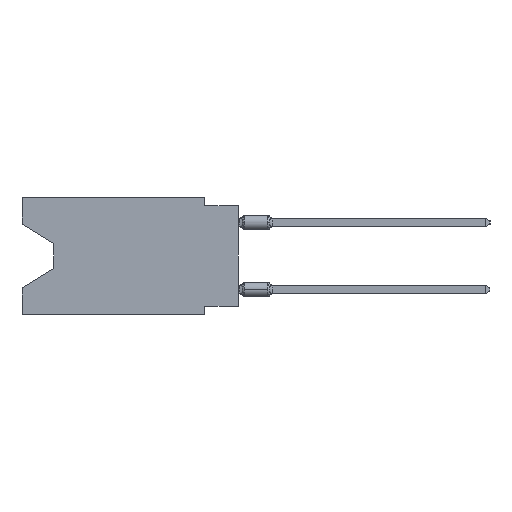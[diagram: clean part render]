
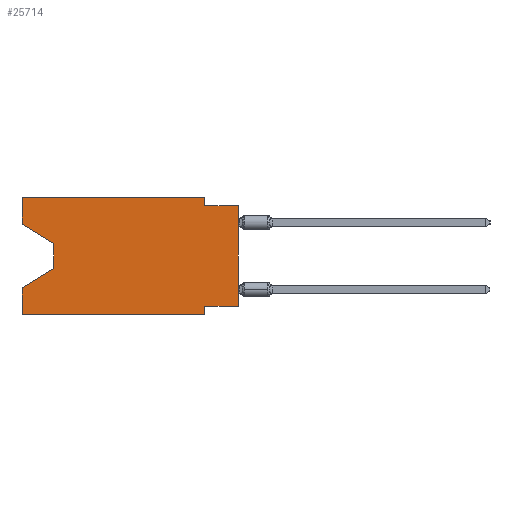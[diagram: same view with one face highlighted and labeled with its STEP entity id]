
A CAD part, left-side view. The second image highlights one B-rep face of the part: STEP entity #25714.
In plain terms, the highlighted planar face has unit normal (-1, 0, 0).
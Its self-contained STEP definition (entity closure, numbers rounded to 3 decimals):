
#379 = AXIS2_PLACEMENT_3D ( 'NONE', #27863, #22950, #36206 ) ;
#764 = DIRECTION ( 'NONE',  ( 0., -1., 0. ) ) ;
#1339 = EDGE_CURVE ( 'NONE', #5638, #7372, #15487, .T. ) ;
#3178 = ORIENTED_EDGE ( 'NONE', *, *, #47952, .F. ) ;
#3217 = VECTOR ( 'NONE', #22056, 1000. ) ;
#4104 = FACE_OUTER_BOUND ( 'NONE', #25687, .T. ) ;
#4354 = LINE ( 'NONE', #56192, #33819 ) ;
#4589 = ORIENTED_EDGE ( 'NONE', *, *, #21904, .T. ) ;
#4931 = EDGE_CURVE ( 'NONE', #29907, #7372, #7942, .T. ) ;
#5638 = VERTEX_POINT ( 'NONE', #30282 ) ;
#6361 = VECTOR ( 'NONE', #45685, 1000. ) ;
#7372 = VERTEX_POINT ( 'NONE', #43385 ) ;
#7942 = LINE ( 'NONE', #41258, #39186 ) ;
#8081 = VERTEX_POINT ( 'NONE', #21407 ) ;
#8949 = CARTESIAN_POINT ( 'NONE',  ( 0., 2.54, -8.89 ) ) ;
#9583 = DIRECTION ( 'NONE',  ( 0., -1., 0. ) ) ;
#10718 = CARTESIAN_POINT ( 'NONE',  ( 0., 0., -0.635 ) ) ;
#10859 = VERTEX_POINT ( 'NONE', #18177 ) ;
#11184 = ORIENTED_EDGE ( 'NONE', *, *, #32861, .F. ) ;
#11634 = DIRECTION ( 'NONE',  ( 0., 0., 1. ) ) ;
#12926 = CARTESIAN_POINT ( 'NONE',  ( 0., 0., 0. ) ) ;
#13536 = DIRECTION ( 'NONE',  ( 0., 0., 1. ) ) ;
#15038 = VECTOR ( 'NONE', #42555, 1000. ) ;
#15487 = LINE ( 'NONE', #20420, #55089 ) ;
#15864 = CARTESIAN_POINT ( 'NONE',  ( 0., 16.383, -8.89 ) ) ;
#16206 = ORIENTED_EDGE ( 'NONE', *, *, #4931, .F. ) ;
#16484 = CARTESIAN_POINT ( 'NONE',  ( 0., 0., -0.635 ) ) ;
#17720 = CARTESIAN_POINT ( 'NONE',  ( 0., 16.383, -2.038 ) ) ;
#17845 = CARTESIAN_POINT ( 'NONE',  ( 0., 0., -8.255 ) ) ;
#18177 = CARTESIAN_POINT ( 'NONE',  ( 0., 2.54, -0.635 ) ) ;
#19493 = VERTEX_POINT ( 'NONE', #24105 ) ;
#19554 = ORIENTED_EDGE ( 'NONE', *, *, #24430, .F. ) ;
#20167 = CARTESIAN_POINT ( 'NONE',  ( 0., 2.54, 0. ) ) ;
#20420 = CARTESIAN_POINT ( 'NONE',  ( 0., 13.97, -5.385 ) ) ;
#20476 = ORIENTED_EDGE ( 'NONE', *, *, #38377, .T. ) ;
#21047 = DIRECTION ( 'NONE',  ( 0., 0.855, -0.519 ) ) ;
#21345 = LINE ( 'NONE', #26259, #6361 ) ;
#21407 = CARTESIAN_POINT ( 'NONE',  ( 0., 2.54, -8.255 ) ) ;
#21811 = LINE ( 'NONE', #53925, #26114 ) ;
#21900 = LINE ( 'NONE', #12926, #53281 ) ;
#21904 = EDGE_CURVE ( 'NONE', #19493, #35493, #21900, .T. ) ;
#22056 = DIRECTION ( 'NONE',  ( 0., -1., 0. ) ) ;
#22950 = DIRECTION ( 'NONE',  ( 1., 0., 0. ) ) ;
#23021 = CARTESIAN_POINT ( 'NONE',  ( 0., 2.54, -8.89 ) ) ;
#23051 = LINE ( 'NONE', #33194, #32774 ) ;
#24105 = CARTESIAN_POINT ( 'NONE',  ( 0., 0., -8.255 ) ) ;
#24430 = EDGE_CURVE ( 'NONE', #10859, #35493, #45185, .T. ) ;
#25687 = EDGE_LOOP ( 'NONE', ( #32043, #39571, #31446, #16206, #20476, #44981, #11184, #4589, #19554, #58121, #3178, #54976 ) ) ;
#25714 = ADVANCED_FACE ( 'NONE', ( #4104 ), #50739, .F. ) ;
#26114 = VECTOR ( 'NONE', #11634, 1000. ) ;
#26259 = CARTESIAN_POINT ( 'NONE',  ( 0., 16.383, -2.038 ) ) ;
#26758 = DIRECTION ( 'NONE',  ( 0., 0., 1. ) ) ;
#27863 = CARTESIAN_POINT ( 'NONE',  ( 0., 16.383, 0. ) ) ;
#28907 = VERTEX_POINT ( 'NONE', #29777 ) ;
#29777 = CARTESIAN_POINT ( 'NONE',  ( 0., 2.54, 0. ) ) ;
#29907 = VERTEX_POINT ( 'NONE', #31164 ) ;
#29924 = VERTEX_POINT ( 'NONE', #59859 ) ;
#30282 = CARTESIAN_POINT ( 'NONE',  ( 0., 13.97, -5.385 ) ) ;
#31164 = CARTESIAN_POINT ( 'NONE',  ( 0., 16.383, -8.89 ) ) ;
#31446 = ORIENTED_EDGE ( 'NONE', *, *, #1339, .T. ) ;
#32043 = ORIENTED_EDGE ( 'NONE', *, *, #39923, .T. ) ;
#32703 = LINE ( 'NONE', #8949, #15038 ) ;
#32774 = VECTOR ( 'NONE', #37816, 1000. ) ;
#32861 = EDGE_CURVE ( 'NONE', #19493, #8081, #60750, .T. ) ;
#33194 = CARTESIAN_POINT ( 'NONE',  ( 0., 13.97, -3.505 ) ) ;
#33819 = VECTOR ( 'NONE', #9583, 1000. ) ;
#35493 = VERTEX_POINT ( 'NONE', #10718 ) ;
#35657 = EDGE_CURVE ( 'NONE', #45273, #37734, #21811, .T. ) ;
#36206 = DIRECTION ( 'NONE',  ( 0., 0., -1. ) ) ;
#36350 = DIRECTION ( 'NONE',  ( 0., 1., 0. ) ) ;
#37734 = VERTEX_POINT ( 'NONE', #58995 ) ;
#37816 = DIRECTION ( 'NONE',  ( 0., 0., -1. ) ) ;
#38250 = VERTEX_POINT ( 'NONE', #23021 ) ;
#38377 = EDGE_CURVE ( 'NONE', #29907, #38250, #58164, .T. ) ;
#39186 = VECTOR ( 'NONE', #26758, 1000. ) ;
#39571 = ORIENTED_EDGE ( 'NONE', *, *, #44199, .T. ) ;
#39923 = EDGE_CURVE ( 'NONE', #45273, #29924, #21345, .T. ) ;
#41258 = CARTESIAN_POINT ( 'NONE',  ( 0., 16.383, 0. ) ) ;
#42555 = DIRECTION ( 'NONE',  ( 0., 0., -1. ) ) ;
#43385 = CARTESIAN_POINT ( 'NONE',  ( 0., 16.383, -6.852 ) ) ;
#44199 = EDGE_CURVE ( 'NONE', #29924, #5638, #23051, .T. ) ;
#44981 = ORIENTED_EDGE ( 'NONE', *, *, #56036, .F. ) ;
#45185 = LINE ( 'NONE', #16484, #3217 ) ;
#45273 = VERTEX_POINT ( 'NONE', #17720 ) ;
#45685 = DIRECTION ( 'NONE',  ( 0., -0.855, -0.519 ) ) ;
#47952 = EDGE_CURVE ( 'NONE', #37734, #28907, #4354, .T. ) ;
#49040 = VECTOR ( 'NONE', #764, 1000. ) ;
#50696 = VECTOR ( 'NONE', #52601, 1000. ) ;
#50739 = PLANE ( 'NONE',  #379 ) ;
#52601 = DIRECTION ( 'NONE',  ( 0., 0., -1. ) ) ;
#52849 = EDGE_CURVE ( 'NONE', #28907, #10859, #53809, .T. ) ;
#53281 = VECTOR ( 'NONE', #13536, 1000. ) ;
#53809 = LINE ( 'NONE', #20167, #50696 ) ;
#53925 = CARTESIAN_POINT ( 'NONE',  ( 0., 16.383, 0. ) ) ;
#54976 = ORIENTED_EDGE ( 'NONE', *, *, #35657, .F. ) ;
#55064 = VECTOR ( 'NONE', #36350, 1000. ) ;
#55089 = VECTOR ( 'NONE', #21047, 1000. ) ;
#56036 = EDGE_CURVE ( 'NONE', #8081, #38250, #32703, .T. ) ;
#56192 = CARTESIAN_POINT ( 'NONE',  ( 0., 16.383, 0. ) ) ;
#58121 = ORIENTED_EDGE ( 'NONE', *, *, #52849, .F. ) ;
#58164 = LINE ( 'NONE', #15864, #49040 ) ;
#58995 = CARTESIAN_POINT ( 'NONE',  ( 0., 16.383, 0. ) ) ;
#59859 = CARTESIAN_POINT ( 'NONE',  ( 0., 13.97, -3.505 ) ) ;
#60750 = LINE ( 'NONE', #17845, #55064 ) ;
